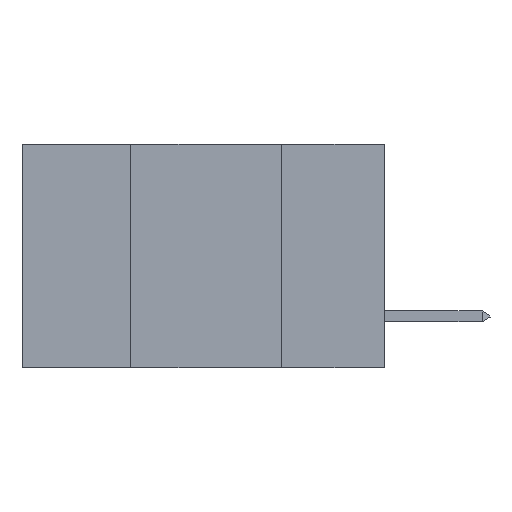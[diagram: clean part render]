
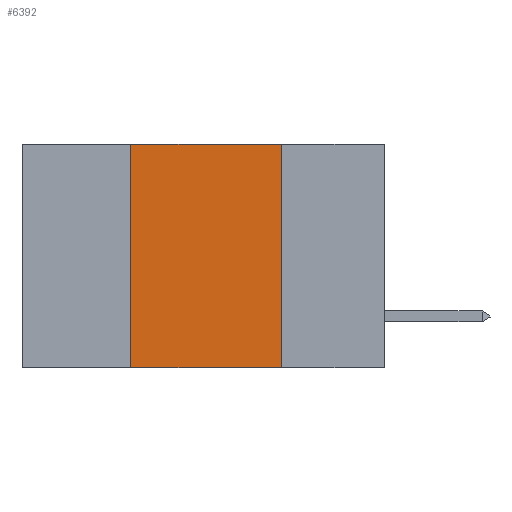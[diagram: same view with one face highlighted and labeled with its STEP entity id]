
A CAD part, left-side view. The second image highlights one B-rep face of the part: STEP entity #6392.
In plain terms, the highlighted planar face has unit normal (-1, 0, 0).
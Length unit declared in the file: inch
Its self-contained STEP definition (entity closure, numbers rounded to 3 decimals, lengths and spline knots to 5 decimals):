
#762 = DIRECTION ( 'NONE',  ( 0., 0., 1. ) ) ;
#818 = VERTEX_POINT ( 'NONE', #12251 ) ;
#850 = ORIENTED_EDGE ( 'NONE', *, *, #5665, .F. ) ;
#1033 = ORIENTED_EDGE ( 'NONE', *, *, #4081, .T. ) ;
#1373 = EDGE_CURVE ( 'NONE', #10862, #13680, #12920, .T. ) ;
#1423 = VECTOR ( 'NONE', #7892, 39.37008 ) ;
#1483 = CARTESIAN_POINT ( 'NONE',  ( 0., 0.17, 0. ) ) ;
#1608 = ORIENTED_EDGE ( 'NONE', *, *, #3789, .F. ) ;
#2542 = CARTESIAN_POINT ( 'NONE',  ( 0., 0.42, 0. ) ) ;
#2769 = VECTOR ( 'NONE', #762, 39.37008 ) ;
#2783 = EDGE_LOOP ( 'NONE', ( #850, #7736, #1608, #1033 ) ) ;
#2998 = VERTEX_POINT ( 'NONE', #12167 ) ;
#3789 = EDGE_CURVE ( 'NONE', #818, #10862, #5977, .T. ) ;
#3959 = CARTESIAN_POINT ( 'NONE',  ( 0., 0.6, 0. ) ) ;
#4081 = EDGE_CURVE ( 'NONE', #818, #2998, #11005, .T. ) ;
#5399 = CARTESIAN_POINT ( 'NONE',  ( 0., 0.6, 0. ) ) ;
#5665 = EDGE_CURVE ( 'NONE', #13680, #2998, #10164, .T. ) ;
#5977 = LINE ( 'NONE', #2542, #2769 ) ;
#6106 = DIRECTION ( 'NONE',  ( 0., 0., -1. ) ) ;
#6392 = ADVANCED_FACE ( 'NONE', ( #7297 ), #10540, .F. ) ;
#6480 = CARTESIAN_POINT ( 'NONE',  ( 0., 0.42, 0. ) ) ;
#6926 = DIRECTION ( 'NONE',  ( 0., -1., 0. ) ) ;
#7297 = FACE_OUTER_BOUND ( 'NONE', #2783, .T. ) ;
#7366 = DIRECTION ( 'NONE',  ( 1., 0., 0. ) ) ;
#7736 = ORIENTED_EDGE ( 'NONE', *, *, #1373, .F. ) ;
#7892 = DIRECTION ( 'NONE',  ( 0., 0., -1. ) ) ;
#8767 = DIRECTION ( 'NONE',  ( 0., -1., 0. ) ) ;
#9859 = VECTOR ( 'NONE', #6926, 39.37008 ) ;
#10164 = LINE ( 'NONE', #1483, #1423 ) ;
#10416 = CARTESIAN_POINT ( 'NONE',  ( 0., 0.17, 0. ) ) ;
#10540 = PLANE ( 'NONE',  #11906 ) ;
#10862 = VERTEX_POINT ( 'NONE', #6480 ) ;
#11005 = LINE ( 'NONE', #11269, #9859 ) ;
#11269 = CARTESIAN_POINT ( 'NONE',  ( 0., 0.6, -0.37 ) ) ;
#11701 = VECTOR ( 'NONE', #8767, 39.37008 ) ;
#11906 = AXIS2_PLACEMENT_3D ( 'NONE', #3959, #7366, #6106 ) ;
#12167 = CARTESIAN_POINT ( 'NONE',  ( 0., 0.17, -0.37 ) ) ;
#12251 = CARTESIAN_POINT ( 'NONE',  ( 0., 0.42, -0.37 ) ) ;
#12920 = LINE ( 'NONE', #5399, #11701 ) ;
#13680 = VERTEX_POINT ( 'NONE', #10416 ) ;
